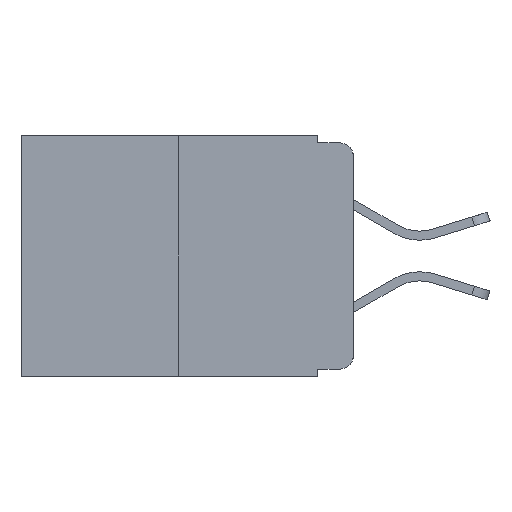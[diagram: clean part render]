
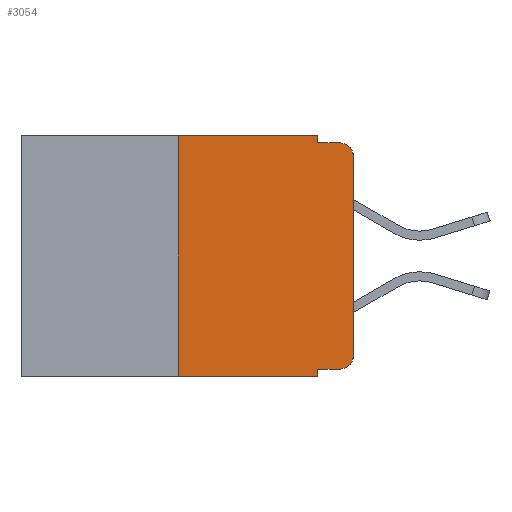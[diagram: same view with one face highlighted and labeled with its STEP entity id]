
A CAD part, left-side view. The second image highlights one B-rep face of the part: STEP entity #3054.
In plain terms, the highlighted planar face has unit normal (-1, 0, 0).
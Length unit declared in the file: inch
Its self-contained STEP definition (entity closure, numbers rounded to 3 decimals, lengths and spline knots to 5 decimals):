
#168 = CARTESIAN_POINT ( 'NONE',  ( 0., 0.02, -0.333 ) ) ;
#192 = EDGE_CURVE ( 'NONE', #10245, #8701, #4354, .T. ) ;
#269 = ORIENTED_EDGE ( 'NONE', *, *, #1795, .T. ) ;
#521 = ORIENTED_EDGE ( 'NONE', *, *, #4739, .F. ) ;
#552 = LINE ( 'NONE', #8346, #8529 ) ;
#737 = FACE_OUTER_BOUND ( 'NONE', #12483, .T. ) ;
#961 = EDGE_CURVE ( 'NONE', #9438, #1860, #7750, .T. ) ;
#1174 = VERTEX_POINT ( 'NONE', #11115 ) ;
#1219 = DIRECTION ( 'NONE',  ( -1., 0., 0. ) ) ;
#1644 = DIRECTION ( 'NONE',  ( 1., 0., 0. ) ) ;
#1653 = DIRECTION ( 'NONE',  ( 0., -1., 0. ) ) ;
#1722 = VECTOR ( 'NONE', #9703, 39.37008 ) ;
#1795 = EDGE_CURVE ( 'NONE', #4541, #1174, #11579, .T. ) ;
#1858 = CARTESIAN_POINT ( 'NONE',  ( 0., 0.051, -0.343 ) ) ;
#1860 = VERTEX_POINT ( 'NONE', #1858 ) ;
#1895 = ORIENTED_EDGE ( 'NONE', *, *, #6552, .F. ) ;
#1943 = CARTESIAN_POINT ( 'NONE',  ( 0., 0.473, 0. ) ) ;
#2074 = VECTOR ( 'NONE', #6464, 39.37008 ) ;
#2087 = DIRECTION ( 'NONE',  ( 0., 0., -1. ) ) ;
#2158 = CARTESIAN_POINT ( 'NONE',  ( 0., 0.25, 0. ) ) ;
#2215 = EDGE_CURVE ( 'NONE', #9438, #4541, #552, .T. ) ;
#2383 = CARTESIAN_POINT ( 'NONE',  ( 0., 0.02, -0.03 ) ) ;
#2663 = CARTESIAN_POINT ( 'NONE',  ( 0., 0.051, -0.01 ) ) ;
#3019 = ORIENTED_EDGE ( 'NONE', *, *, #11200, .T. ) ;
#3054 = ADVANCED_FACE ( 'NONE', ( #737 ), #10506, .F. ) ;
#3211 = DIRECTION ( 'NONE',  ( 0., 0., -1. ) ) ;
#3337 = LINE ( 'NONE', #8940, #8151 ) ;
#3425 = VERTEX_POINT ( 'NONE', #2663 ) ;
#3722 = ORIENTED_EDGE ( 'NONE', *, *, #2215, .T. ) ;
#3757 = ORIENTED_EDGE ( 'NONE', *, *, #192, .T. ) ;
#3786 = LINE ( 'NONE', #12525, #7093 ) ;
#3848 = DIRECTION ( 'NONE',  ( 0., 0., -1. ) ) ;
#4270 = AXIS2_PLACEMENT_3D ( 'NONE', #10434, #1644, #11467 ) ;
#4291 = VERTEX_POINT ( 'NONE', #10509 ) ;
#4354 = CIRCLE ( 'NONE', #11482, 0.02 ) ;
#4541 = VERTEX_POINT ( 'NONE', #168 ) ;
#4625 = LINE ( 'NONE', #5627, #2074 ) ;
#4739 = EDGE_CURVE ( 'NONE', #7601, #4291, #12035, .T. ) ;
#5316 = CARTESIAN_POINT ( 'NONE',  ( 0., 0.051, 0. ) ) ;
#5564 = EDGE_CURVE ( 'NONE', #1174, #10245, #3337, .T. ) ;
#5627 = CARTESIAN_POINT ( 'NONE',  ( 0., 0.051, -0.01 ) ) ;
#5682 = VECTOR ( 'NONE', #2087, 39.37008 ) ;
#5769 = ORIENTED_EDGE ( 'NONE', *, *, #961, .F. ) ;
#5882 = ORIENTED_EDGE ( 'NONE', *, *, #7203, .F. ) ;
#5885 = LINE ( 'NONE', #1943, #1722 ) ;
#6028 = DIRECTION ( 'NONE',  ( 0., 0., 1. ) ) ;
#6405 = CARTESIAN_POINT ( 'NONE',  ( 0., 0.473, -0.343 ) ) ;
#6445 = VERTEX_POINT ( 'NONE', #5316 ) ;
#6464 = DIRECTION ( 'NONE',  ( 0., -1., 0. ) ) ;
#6523 = LINE ( 'NONE', #6405, #7606 ) ;
#6552 = EDGE_CURVE ( 'NONE', #3425, #8701, #4625, .T. ) ;
#6850 = CARTESIAN_POINT ( 'NONE',  ( 0., 0.02, -0.313 ) ) ;
#7093 = VECTOR ( 'NONE', #3848, 39.37008 ) ;
#7203 = EDGE_CURVE ( 'NONE', #6445, #3425, #3786, .T. ) ;
#7601 = VERTEX_POINT ( 'NONE', #8295 ) ;
#7606 = VECTOR ( 'NONE', #10343, 39.37008 ) ;
#7750 = LINE ( 'NONE', #8009, #5682 ) ;
#8009 = CARTESIAN_POINT ( 'NONE',  ( 0., 0.051, 0. ) ) ;
#8151 = VECTOR ( 'NONE', #10911, 39.37008 ) ;
#8169 = ORIENTED_EDGE ( 'NONE', *, *, #5564, .T. ) ;
#8295 = CARTESIAN_POINT ( 'NONE',  ( 0., 0.25, -0.343 ) ) ;
#8346 = CARTESIAN_POINT ( 'NONE',  ( 0., 0.051, -0.333 ) ) ;
#8529 = VECTOR ( 'NONE', #1653, 39.37008 ) ;
#8701 = VERTEX_POINT ( 'NONE', #8880 ) ;
#8753 = VECTOR ( 'NONE', #6028, 39.37008 ) ;
#8810 = DIRECTION ( 'NONE',  ( -1., 0., 0. ) ) ;
#8856 = CARTESIAN_POINT ( 'NONE',  ( 0., 0.051, -0.333 ) ) ;
#8880 = CARTESIAN_POINT ( 'NONE',  ( 0., 0.02, -0.01 ) ) ;
#8940 = CARTESIAN_POINT ( 'NONE',  ( 0., 0., 0. ) ) ;
#9438 = VERTEX_POINT ( 'NONE', #8856 ) ;
#9703 = DIRECTION ( 'NONE',  ( 0., -1., 0. ) ) ;
#10245 = VERTEX_POINT ( 'NONE', #10481 ) ;
#10335 = AXIS2_PLACEMENT_3D ( 'NONE', #6850, #8810, #11688 ) ;
#10343 = DIRECTION ( 'NONE',  ( 0., -1., 0. ) ) ;
#10434 = CARTESIAN_POINT ( 'NONE',  ( 0., 0.473, 0. ) ) ;
#10481 = CARTESIAN_POINT ( 'NONE',  ( 0., 0., -0.03 ) ) ;
#10506 = PLANE ( 'NONE',  #4270 ) ;
#10509 = CARTESIAN_POINT ( 'NONE',  ( 0., 0.25, 0. ) ) ;
#10911 = DIRECTION ( 'NONE',  ( 0., 0., 1. ) ) ;
#11115 = CARTESIAN_POINT ( 'NONE',  ( 0., 0., -0.313 ) ) ;
#11200 = EDGE_CURVE ( 'NONE', #7601, #1860, #6523, .T. ) ;
#11411 = EDGE_CURVE ( 'NONE', #4291, #6445, #5885, .T. ) ;
#11467 = DIRECTION ( 'NONE',  ( 0., 0., -1. ) ) ;
#11482 = AXIS2_PLACEMENT_3D ( 'NONE', #2383, #1219, #3211 ) ;
#11579 = CIRCLE ( 'NONE', #10335, 0.02 ) ;
#11688 = DIRECTION ( 'NONE',  ( 0., 0., -1. ) ) ;
#12035 = LINE ( 'NONE', #2158, #8753 ) ;
#12483 = EDGE_LOOP ( 'NONE', ( #8169, #3757, #1895, #5882, #12571, #521, #3019, #5769, #3722, #269 ) ) ;
#12525 = CARTESIAN_POINT ( 'NONE',  ( 0., 0.051, 0. ) ) ;
#12571 = ORIENTED_EDGE ( 'NONE', *, *, #11411, .F. ) ;
